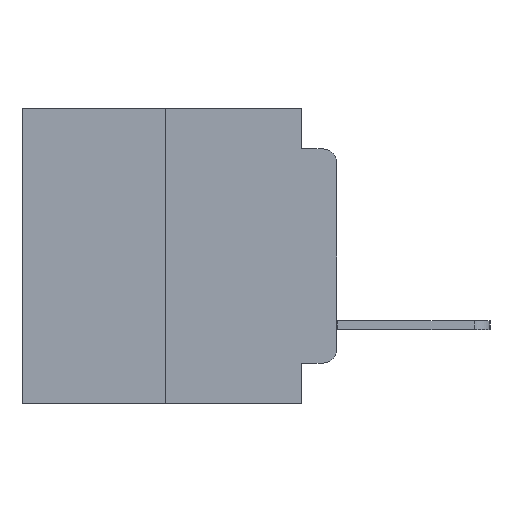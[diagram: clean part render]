
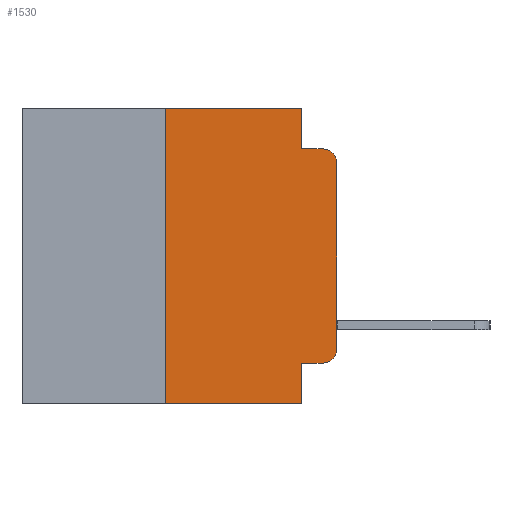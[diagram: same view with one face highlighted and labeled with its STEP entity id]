
A CAD part, left-side view. The second image highlights one B-rep face of the part: STEP entity #1530.
In plain terms, the highlighted planar face has unit normal (-1, 0, 0).
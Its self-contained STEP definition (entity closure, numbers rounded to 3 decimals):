
#6 = ORIENTED_EDGE ( 'NONE', *, *, #2755, .F. ) ;
#180 = DIRECTION ( 'NONE',  ( 0., -1., 0. ) ) ;
#674 = VERTEX_POINT ( 'NONE', #16100 ) ;
#733 = VERTEX_POINT ( 'NONE', #12151 ) ;
#1263 = EDGE_CURVE ( 'NONE', #25468, #12356, #14403, .T. ) ;
#1530 = ADVANCED_FACE ( 'NONE', ( #27747 ), #3472, .F. ) ;
#1685 = EDGE_CURVE ( 'NONE', #12350, #733, #14735, .T. ) ;
#1815 = DIRECTION ( 'NONE',  ( 0., 0., -1. ) ) ;
#1939 = ORIENTED_EDGE ( 'NONE', *, *, #1685, .T. ) ;
#2394 = AXIS2_PLACEMENT_3D ( 'NONE', #25951, #4241, #21365 ) ;
#2755 = EDGE_CURVE ( 'NONE', #3910, #12114, #22227, .T. ) ;
#3472 = PLANE ( 'NONE',  #22791 ) ;
#3540 = ORIENTED_EDGE ( 'NONE', *, *, #1263, .T. ) ;
#3548 = VECTOR ( 'NONE', #14080, 1000. ) ;
#3822 = CARTESIAN_POINT ( 'NONE',  ( -75.603, 11.684, -5.486 ) ) ;
#3905 = CARTESIAN_POINT ( 'NONE',  ( -75.603, 1.295, 0. ) ) ;
#3910 = VERTEX_POINT ( 'NONE', #21358 ) ;
#4189 = DIRECTION ( 'NONE',  ( 1., 0., 0. ) ) ;
#4241 = DIRECTION ( 'NONE',  ( -1., 0., 0. ) ) ;
#4264 = VERTEX_POINT ( 'NONE', #17504 ) ;
#4425 = EDGE_CURVE ( 'NONE', #26079, #20761, #23984, .T. ) ;
#6446 = CIRCLE ( 'NONE', #20917, 0.508 ) ;
#6528 = CARTESIAN_POINT ( 'NONE',  ( -75.603, 0.508, 3.467 ) ) ;
#7512 = VECTOR ( 'NONE', #26881, 1000. ) ;
#7539 = VECTOR ( 'NONE', #17272, 1000. ) ;
#7583 = CARTESIAN_POINT ( 'NONE',  ( -75.603, 1.295, 0. ) ) ;
#7660 = VECTOR ( 'NONE', #1815, 1000. ) ;
#8031 = ORIENTED_EDGE ( 'NONE', *, *, #24205, .F. ) ;
#8309 = LINE ( 'NONE', #13056, #25084 ) ;
#8470 = LINE ( 'NONE', #12002, #14976 ) ;
#8920 = DIRECTION ( 'NONE',  ( 0., -1., 0. ) ) ;
#8930 = DIRECTION ( 'NONE',  ( -1., 0., 0. ) ) ;
#9357 = LINE ( 'NONE', #7583, #3548 ) ;
#9574 = CARTESIAN_POINT ( 'NONE',  ( -75.603, 0., 5.486 ) ) ;
#9610 = ORIENTED_EDGE ( 'NONE', *, *, #18500, .T. ) ;
#10477 = DIRECTION ( 'NONE',  ( 0., 0., -1. ) ) ;
#11177 = ORIENTED_EDGE ( 'NONE', *, *, #26540, .T. ) ;
#11765 = LINE ( 'NONE', #3905, #7660 ) ;
#12002 = CARTESIAN_POINT ( 'NONE',  ( -75.603, 6.35, -5.486 ) ) ;
#12114 = VERTEX_POINT ( 'NONE', #20964 ) ;
#12151 = CARTESIAN_POINT ( 'NONE',  ( -75.603, 0.508, -3.975 ) ) ;
#12350 = VERTEX_POINT ( 'NONE', #23913 ) ;
#12356 = VERTEX_POINT ( 'NONE', #28312 ) ;
#13056 = CARTESIAN_POINT ( 'NONE',  ( -75.603, 11.684, 5.486 ) ) ;
#14080 = DIRECTION ( 'NONE',  ( 0., 0., -1. ) ) ;
#14317 = ORIENTED_EDGE ( 'NONE', *, *, #4425, .T. ) ;
#14403 = LINE ( 'NONE', #3822, #20591 ) ;
#14735 = LINE ( 'NONE', #21500, #7539 ) ;
#14976 = VECTOR ( 'NONE', #27603, 1000. ) ;
#15546 = EDGE_CURVE ( 'NONE', #12350, #12356, #9357, .T. ) ;
#16100 = CARTESIAN_POINT ( 'NONE',  ( -75.603, 1.295, 5.486 ) ) ;
#16416 = ORIENTED_EDGE ( 'NONE', *, *, #21662, .F. ) ;
#17272 = DIRECTION ( 'NONE',  ( 0., -1., 0. ) ) ;
#17504 = CARTESIAN_POINT ( 'NONE',  ( -75.603, 6.35, 5.486 ) ) ;
#17608 = CARTESIAN_POINT ( 'NONE',  ( -75.603, 1.295, 3.975 ) ) ;
#18132 = CARTESIAN_POINT ( 'NONE',  ( -75.603, 0., -3.467 ) ) ;
#18500 = EDGE_CURVE ( 'NONE', #20761, #12114, #6446, .T. ) ;
#19031 = CARTESIAN_POINT ( 'NONE',  ( -75.603, 0., 3.467 ) ) ;
#19320 = ORIENTED_EDGE ( 'NONE', *, *, #15546, .F. ) ;
#19813 = CIRCLE ( 'NONE', #2394, 0.508 ) ;
#19872 = EDGE_CURVE ( 'NONE', #25468, #4264, #8470, .T. ) ;
#20591 = VECTOR ( 'NONE', #23154, 1000. ) ;
#20761 = VERTEX_POINT ( 'NONE', #19031 ) ;
#20917 = AXIS2_PLACEMENT_3D ( 'NONE', #6528, #8930, #26231 ) ;
#20964 = CARTESIAN_POINT ( 'NONE',  ( -75.603, 0.508, 3.975 ) ) ;
#21358 = CARTESIAN_POINT ( 'NONE',  ( -75.603, 1.295, 3.975 ) ) ;
#21365 = DIRECTION ( 'NONE',  ( 0., 0., -1. ) ) ;
#21500 = CARTESIAN_POINT ( 'NONE',  ( -75.603, 1.295, -3.975 ) ) ;
#21662 = EDGE_CURVE ( 'NONE', #674, #3910, #11765, .T. ) ;
#22227 = LINE ( 'NONE', #17608, #25279 ) ;
#22791 = AXIS2_PLACEMENT_3D ( 'NONE', #28286, #4189, #10477 ) ;
#23154 = DIRECTION ( 'NONE',  ( 0., -1., 0. ) ) ;
#23804 = ORIENTED_EDGE ( 'NONE', *, *, #19872, .F. ) ;
#23913 = CARTESIAN_POINT ( 'NONE',  ( -75.603, 1.295, -3.975 ) ) ;
#23984 = LINE ( 'NONE', #9574, #7512 ) ;
#24205 = EDGE_CURVE ( 'NONE', #4264, #674, #8309, .T. ) ;
#25084 = VECTOR ( 'NONE', #180, 1000. ) ;
#25279 = VECTOR ( 'NONE', #8920, 1000. ) ;
#25468 = VERTEX_POINT ( 'NONE', #26484 ) ;
#25794 = EDGE_LOOP ( 'NONE', ( #1939, #11177, #14317, #9610, #6, #16416, #8031, #23804, #3540, #19320 ) ) ;
#25951 = CARTESIAN_POINT ( 'NONE',  ( -75.603, 0.508, -3.467 ) ) ;
#26079 = VERTEX_POINT ( 'NONE', #18132 ) ;
#26231 = DIRECTION ( 'NONE',  ( 0., 0., -1. ) ) ;
#26484 = CARTESIAN_POINT ( 'NONE',  ( -75.603, 6.35, -5.486 ) ) ;
#26540 = EDGE_CURVE ( 'NONE', #733, #26079, #19813, .T. ) ;
#26881 = DIRECTION ( 'NONE',  ( 0., 0., 1. ) ) ;
#27603 = DIRECTION ( 'NONE',  ( 0., 0., 1. ) ) ;
#27747 = FACE_OUTER_BOUND ( 'NONE', #25794, .T. ) ;
#28286 = CARTESIAN_POINT ( 'NONE',  ( -75.603, 11.684, 5.486 ) ) ;
#28312 = CARTESIAN_POINT ( 'NONE',  ( -75.603, 1.295, -5.486 ) ) ;
